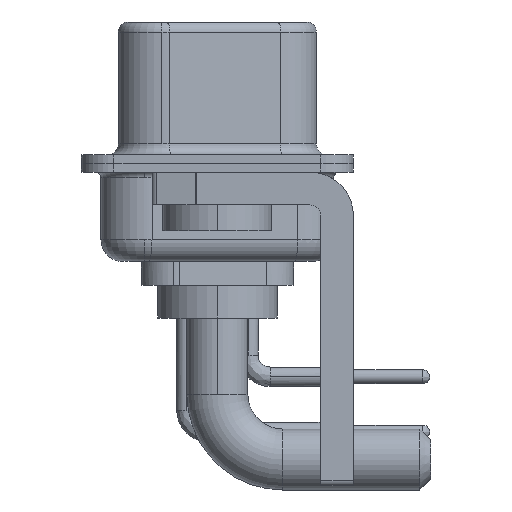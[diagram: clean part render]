
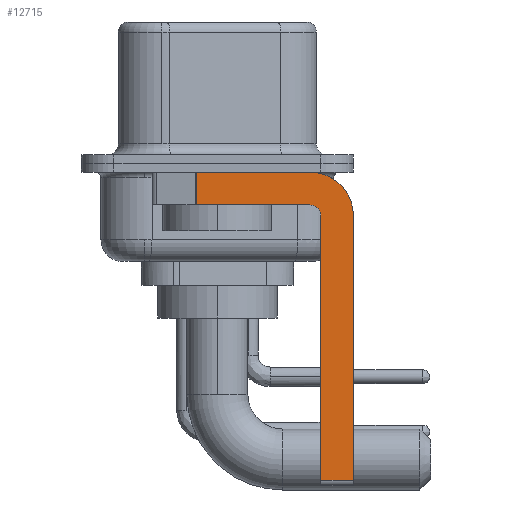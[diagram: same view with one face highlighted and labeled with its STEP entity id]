
A CAD part, left-side view. The second image highlights one B-rep face of the part: STEP entity #12715.
In plain terms, the highlighted planar face has unit normal (-1, 0, 0).
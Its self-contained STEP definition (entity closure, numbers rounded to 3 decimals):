
#675 = ORIENTED_EDGE ( 'NONE', *, *, #21445, .F. ) ;
#969 = ORIENTED_EDGE ( 'NONE', *, *, #24759, .F. ) ;
#1611 = VECTOR ( 'NONE', #11764, 1000. ) ;
#1661 = ORIENTED_EDGE ( 'NONE', *, *, #15094, .F. ) ;
#2020 = EDGE_CURVE ( 'NONE', #18450, #4216, #23175, .T. ) ;
#2140 = VERTEX_POINT ( 'NONE', #9646 ) ;
#2247 = CARTESIAN_POINT ( 'NONE',  ( -2.9, -4.25, -14.55 ) ) ;
#2565 = CARTESIAN_POINT ( 'NONE',  ( -2.9, -6.25, -2.4 ) ) ;
#3014 = ORIENTED_EDGE ( 'NONE', *, *, #12587, .T. ) ;
#3069 = DIRECTION ( 'NONE',  ( 0., -1., 0. ) ) ;
#3248 = CIRCLE ( 'NONE', #8212, 2. ) ;
#3962 = LINE ( 'NONE', #6915, #24189 ) ;
#4197 = LINE ( 'NONE', #2247, #25429 ) ;
#4216 = VERTEX_POINT ( 'NONE', #18155 ) ;
#4792 = VECTOR ( 'NONE', #14348, 1000. ) ;
#5436 = VERTEX_POINT ( 'NONE', #14837 ) ;
#6402 = CARTESIAN_POINT ( 'NONE',  ( -2.9, -4.25, -2.4 ) ) ;
#6532 = DIRECTION ( 'NONE',  ( 1., 0., 0. ) ) ;
#6791 = DIRECTION ( 'NONE',  ( 0., 0., -1. ) ) ;
#6915 = CARTESIAN_POINT ( 'NONE',  ( -2.9, 0.978, -1.9 ) ) ;
#7068 = CARTESIAN_POINT ( 'NONE',  ( -2.9, -4.75, -14.55 ) ) ;
#7394 = DIRECTION ( 'NONE',  ( 0., 0., -1. ) ) ;
#7610 = DIRECTION ( 'NONE',  ( 0., 0., 1. ) ) ;
#7992 = AXIS2_PLACEMENT_3D ( 'NONE', #6402, #6532, #20311 ) ;
#8166 = EDGE_LOOP ( 'NONE', ( #11707, #3014, #22129, #969, #9347, #12534, #1661, #675 ) ) ;
#8212 = AXIS2_PLACEMENT_3D ( 'NONE', #17386, #23111, #7394 ) ;
#8340 = FACE_OUTER_BOUND ( 'NONE', #8166, .T. ) ;
#8351 = CARTESIAN_POINT ( 'NONE',  ( -2.9, -6.25, -2.4 ) ) ;
#9071 = VECTOR ( 'NONE', #3069, 1000. ) ;
#9294 = CARTESIAN_POINT ( 'NONE',  ( -2.9, -4.75, -14.8 ) ) ;
#9347 = ORIENTED_EDGE ( 'NONE', *, *, #19511, .F. ) ;
#9646 = CARTESIAN_POINT ( 'NONE',  ( -2.9, 0.978, -1.9 ) ) ;
#10790 = CARTESIAN_POINT ( 'NONE',  ( -2.9, 0.978, -0.4 ) ) ;
#10839 = EDGE_CURVE ( 'NONE', #23783, #13271, #4197, .T. ) ;
#11383 = CARTESIAN_POINT ( 'NONE',  ( -2.9, -4.25, -1.9 ) ) ;
#11707 = ORIENTED_EDGE ( 'NONE', *, *, #2020, .F. ) ;
#11764 = DIRECTION ( 'NONE',  ( 0., 1., 0. ) ) ;
#12267 = LINE ( 'NONE', #8351, #4792 ) ;
#12534 = ORIENTED_EDGE ( 'NONE', *, *, #10839, .T. ) ;
#12587 = EDGE_CURVE ( 'NONE', #18450, #2140, #3962, .T. ) ;
#12715 = ADVANCED_FACE ( 'NONE', ( #8340 ), #24197, .F. ) ;
#13271 = VERTEX_POINT ( 'NONE', #15286 ) ;
#14348 = DIRECTION ( 'NONE',  ( 0., 0., -1. ) ) ;
#14837 = CARTESIAN_POINT ( 'NONE',  ( -2.9, -4.25, -1.9 ) ) ;
#15094 = EDGE_CURVE ( 'NONE', #19288, #13271, #12267, .T. ) ;
#15153 = CARTESIAN_POINT ( 'NONE',  ( -2.9, -4.25, -2.4 ) ) ;
#15286 = CARTESIAN_POINT ( 'NONE',  ( -2.9, -6.25, -14.55 ) ) ;
#15526 = LINE ( 'NONE', #9294, #23574 ) ;
#16684 = CIRCLE ( 'NONE', #24558, 0.5 ) ;
#16847 = DIRECTION ( 'NONE',  ( -1., 0., 0. ) ) ;
#17386 = CARTESIAN_POINT ( 'NONE',  ( -2.9, -4.25, -2.4 ) ) ;
#18155 = CARTESIAN_POINT ( 'NONE',  ( -2.9, -4.25, -0.4 ) ) ;
#18450 = VERTEX_POINT ( 'NONE', #10790 ) ;
#18690 = DIRECTION ( 'NONE',  ( 0., 0., 1. ) ) ;
#19288 = VERTEX_POINT ( 'NONE', #2565 ) ;
#19418 = CARTESIAN_POINT ( 'NONE',  ( -2.9, 3., -0.4 ) ) ;
#19439 = LINE ( 'NONE', #11383, #1611 ) ;
#19484 = CARTESIAN_POINT ( 'NONE',  ( -2.9, -4.75, -2.4 ) ) ;
#19511 = EDGE_CURVE ( 'NONE', #23783, #21433, #15526, .T. ) ;
#19632 = EDGE_CURVE ( 'NONE', #5436, #2140, #19439, .T. ) ;
#20311 = DIRECTION ( 'NONE',  ( 0., 0., -1. ) ) ;
#21433 = VERTEX_POINT ( 'NONE', #19484 ) ;
#21445 = EDGE_CURVE ( 'NONE', #4216, #19288, #3248, .T. ) ;
#22129 = ORIENTED_EDGE ( 'NONE', *, *, #19632, .F. ) ;
#23111 = DIRECTION ( 'NONE',  ( 1., 0., 0. ) ) ;
#23175 = LINE ( 'NONE', #19418, #9071 ) ;
#23574 = VECTOR ( 'NONE', #7610, 1000. ) ;
#23783 = VERTEX_POINT ( 'NONE', #7068 ) ;
#23928 = DIRECTION ( 'NONE',  ( 0., -1., 0. ) ) ;
#24189 = VECTOR ( 'NONE', #6791, 1000. ) ;
#24197 = PLANE ( 'NONE',  #7992 ) ;
#24558 = AXIS2_PLACEMENT_3D ( 'NONE', #15153, #16847, #18690 ) ;
#24759 = EDGE_CURVE ( 'NONE', #21433, #5436, #16684, .T. ) ;
#25429 = VECTOR ( 'NONE', #23928, 1000. ) ;
